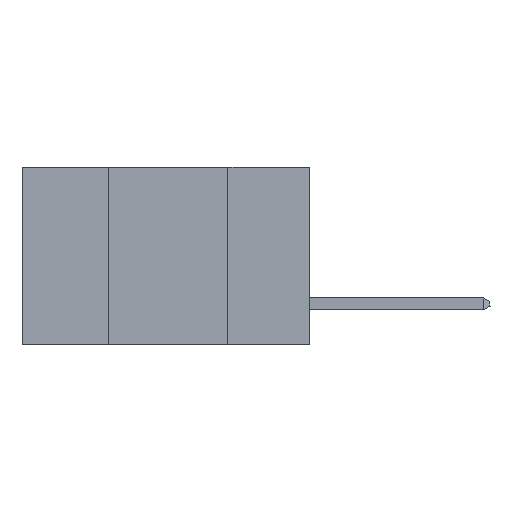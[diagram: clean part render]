
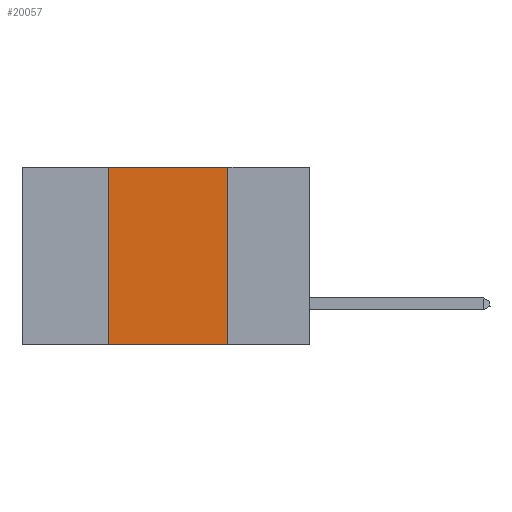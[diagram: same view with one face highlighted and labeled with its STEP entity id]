
A CAD part, left-side view. The second image highlights one B-rep face of the part: STEP entity #20057.
In plain terms, the highlighted planar face has unit normal (-1, 0, 0).
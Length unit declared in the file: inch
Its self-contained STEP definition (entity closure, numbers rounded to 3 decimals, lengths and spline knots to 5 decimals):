
#792 = DIRECTION ( 'NONE',  ( 0., -1., 0. ) ) ;
#1243 = VERTEX_POINT ( 'NONE', #22805 ) ;
#1312 = ORIENTED_EDGE ( 'NONE', *, *, #13495, .F. ) ;
#1535 = CARTESIAN_POINT ( 'NONE',  ( 0., 0.42, -0.37 ) ) ;
#2389 = LINE ( 'NONE', #17087, #5842 ) ;
#3844 = EDGE_CURVE ( 'NONE', #17728, #11522, #13433, .T. ) ;
#3898 = VERTEX_POINT ( 'NONE', #10561 ) ;
#4500 = VECTOR ( 'NONE', #14937, 39.37008 ) ;
#5204 = CARTESIAN_POINT ( 'NONE',  ( 0., 0.42, 0. ) ) ;
#5842 = VECTOR ( 'NONE', #15220, 39.37008 ) ;
#8404 = LINE ( 'NONE', #14872, #18994 ) ;
#9894 = ORIENTED_EDGE ( 'NONE', *, *, #3844, .T. ) ;
#10442 = LINE ( 'NONE', #5204, #15958 ) ;
#10561 = CARTESIAN_POINT ( 'NONE',  ( 0., 0.42, 0. ) ) ;
#11522 = VERTEX_POINT ( 'NONE', #22980 ) ;
#12518 = ORIENTED_EDGE ( 'NONE', *, *, #14302, .F. ) ;
#13433 = LINE ( 'NONE', #15099, #4500 ) ;
#13495 = EDGE_CURVE ( 'NONE', #17728, #3898, #10442, .T. ) ;
#14302 = EDGE_CURVE ( 'NONE', #3898, #1243, #8404, .T. ) ;
#14872 = CARTESIAN_POINT ( 'NONE',  ( 0., 0.6, 0. ) ) ;
#14937 = DIRECTION ( 'NONE',  ( 0., -1., 0. ) ) ;
#15045 = DIRECTION ( 'NONE',  ( 0., 0., -1. ) ) ;
#15099 = CARTESIAN_POINT ( 'NONE',  ( 0., 0.6, -0.37 ) ) ;
#15220 = DIRECTION ( 'NONE',  ( 0., 0., -1. ) ) ;
#15337 = AXIS2_PLACEMENT_3D ( 'NONE', #18953, #15363, #15045 ) ;
#15363 = DIRECTION ( 'NONE',  ( 1., 0., 0. ) ) ;
#15763 = FACE_OUTER_BOUND ( 'NONE', #21696, .T. ) ;
#15958 = VECTOR ( 'NONE', #19375, 39.37008 ) ;
#17087 = CARTESIAN_POINT ( 'NONE',  ( 0., 0.17, 0. ) ) ;
#17589 = EDGE_CURVE ( 'NONE', #1243, #11522, #2389, .T. ) ;
#17728 = VERTEX_POINT ( 'NONE', #1535 ) ;
#18710 = PLANE ( 'NONE',  #15337 ) ;
#18902 = ORIENTED_EDGE ( 'NONE', *, *, #17589, .F. ) ;
#18953 = CARTESIAN_POINT ( 'NONE',  ( 0., 0.6, 0. ) ) ;
#18994 = VECTOR ( 'NONE', #792, 39.37008 ) ;
#19375 = DIRECTION ( 'NONE',  ( 0., 0., 1. ) ) ;
#20057 = ADVANCED_FACE ( 'NONE', ( #15763 ), #18710, .F. ) ;
#21696 = EDGE_LOOP ( 'NONE', ( #18902, #12518, #1312, #9894 ) ) ;
#22805 = CARTESIAN_POINT ( 'NONE',  ( 0., 0.17, 0. ) ) ;
#22980 = CARTESIAN_POINT ( 'NONE',  ( 0., 0.17, -0.37 ) ) ;
